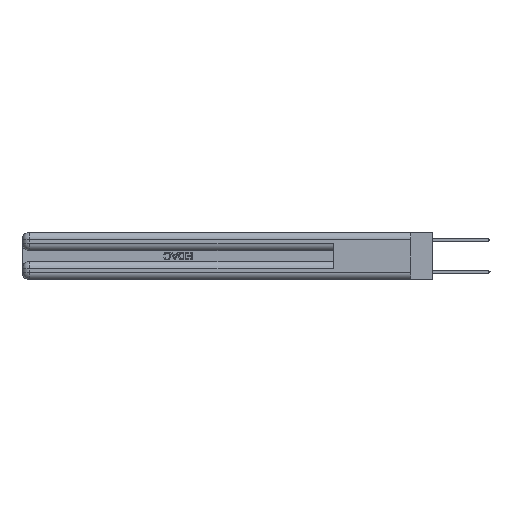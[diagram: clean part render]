
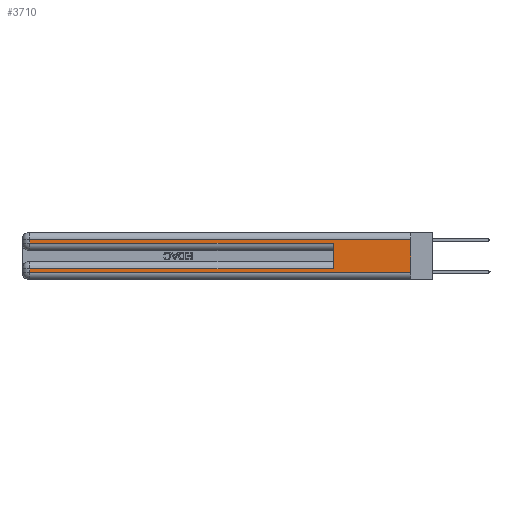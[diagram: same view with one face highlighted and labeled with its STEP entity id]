
A CAD part, left-side view. The second image highlights one B-rep face of the part: STEP entity #3710.
In plain terms, the highlighted planar face has unit normal (-1, 0, 0).
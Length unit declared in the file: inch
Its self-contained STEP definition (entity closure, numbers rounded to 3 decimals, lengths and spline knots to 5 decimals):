
#791 = EDGE_CURVE ( 'NONE', #13586, #18417, #19519, .T. ) ;
#1334 = CARTESIAN_POINT ( 'NONE',  ( 0., 2.94, 0.37 ) ) ;
#1484 = VECTOR ( 'NONE', #6819, 39.37008 ) ;
#2397 = PLANE ( 'NONE',  #27314 ) ;
#2539 = VECTOR ( 'NONE', #17491, 39.37008 ) ;
#3710 = ADVANCED_FACE ( 'NONE', ( #32501 ), #2397, .F. ) ;
#4244 = VERTEX_POINT ( 'NONE', #26098 ) ;
#4618 = ORIENTED_EDGE ( 'NONE', *, *, #24827, .T. ) ;
#5021 = ORIENTED_EDGE ( 'NONE', *, *, #18827, .T. ) ;
#5046 = VECTOR ( 'NONE', #24689, 39.37008 ) ;
#5087 = CARTESIAN_POINT ( 'NONE',  ( 0., 0., 0.37 ) ) ;
#5251 = VECTOR ( 'NONE', #16092, 39.37008 ) ;
#5774 = ORIENTED_EDGE ( 'NONE', *, *, #29402, .F. ) ;
#5963 = ORIENTED_EDGE ( 'NONE', *, *, #29117, .T. ) ;
#6102 = CARTESIAN_POINT ( 'NONE',  ( 0., 0., 0.285 ) ) ;
#6352 = VECTOR ( 'NONE', #8772, 39.37008 ) ;
#6819 = DIRECTION ( 'NONE',  ( 0., 0., -1. ) ) ;
#7538 = CARTESIAN_POINT ( 'NONE',  ( 0., 0., 0.06 ) ) ;
#7709 = ORIENTED_EDGE ( 'NONE', *, *, #9601, .T. ) ;
#7748 = CARTESIAN_POINT ( 'NONE',  ( 0., 0.6, 0.285 ) ) ;
#7762 = DIRECTION ( 'NONE',  ( 0., 0., -1. ) ) ;
#8162 = DIRECTION ( 'NONE',  ( 0., 0., 1. ) ) ;
#8569 = LINE ( 'NONE', #1334, #1484 ) ;
#8772 = DIRECTION ( 'NONE',  ( 0., -1., 0. ) ) ;
#8847 = CARTESIAN_POINT ( 'NONE',  ( 0., 0., 0.31 ) ) ;
#8966 = VECTOR ( 'NONE', #30380, 39.37008 ) ;
#9601 = EDGE_CURVE ( 'NONE', #30058, #17965, #8569, .T. ) ;
#9662 = LINE ( 'NONE', #27959, #2539 ) ;
#10101 = ORIENTED_EDGE ( 'NONE', *, *, #791, .F. ) ;
#10317 = ORIENTED_EDGE ( 'NONE', *, *, #25605, .T. ) ;
#10763 = CARTESIAN_POINT ( 'NONE',  ( 0., 0., 0.085 ) ) ;
#10765 = VERTEX_POINT ( 'NONE', #7538 ) ;
#10794 = DIRECTION ( 'NONE',  ( 0., 0., -1. ) ) ;
#11095 = CARTESIAN_POINT ( 'NONE',  ( 0., 0.6, 0.085 ) ) ;
#12100 = CARTESIAN_POINT ( 'NONE',  ( 0., 2.94, 0.31 ) ) ;
#12458 = VECTOR ( 'NONE', #8162, 39.37008 ) ;
#12657 = LINE ( 'NONE', #23965, #26691 ) ;
#13227 = CARTESIAN_POINT ( 'NONE',  ( 0., 2.94, 0.085 ) ) ;
#13402 = LINE ( 'NONE', #6102, #6352 ) ;
#13586 = VERTEX_POINT ( 'NONE', #11095 ) ;
#13772 = LINE ( 'NONE', #8847, #5046 ) ;
#16092 = DIRECTION ( 'NONE',  ( 0., 1., 0. ) ) ;
#17491 = DIRECTION ( 'NONE',  ( 0., -1., 0. ) ) ;
#17965 = VERTEX_POINT ( 'NONE', #26971 ) ;
#18017 = CARTESIAN_POINT ( 'NONE',  ( 0., 0., 0.31 ) ) ;
#18417 = VERTEX_POINT ( 'NONE', #7748 ) ;
#18827 = EDGE_CURVE ( 'NONE', #4244, #10765, #9662, .T. ) ;
#18851 = CARTESIAN_POINT ( 'NONE',  ( 0., 0.6, 0.145 ) ) ;
#19519 = LINE ( 'NONE', #18851, #12458 ) ;
#21656 = ORIENTED_EDGE ( 'NONE', *, *, #24171, .T. ) ;
#22458 = EDGE_LOOP ( 'NONE', ( #5774, #10317, #7709, #4618, #10101, #5963, #21656, #5021 ) ) ;
#23620 = DIRECTION ( 'NONE',  ( 1., 0., 0. ) ) ;
#23965 = CARTESIAN_POINT ( 'NONE',  ( 0., 2.94, 0.37 ) ) ;
#24171 = EDGE_CURVE ( 'NONE', #30370, #4244, #12657, .T. ) ;
#24689 = DIRECTION ( 'NONE',  ( 0., 1., 0. ) ) ;
#24827 = EDGE_CURVE ( 'NONE', #17965, #18417, #13402, .T. ) ;
#25061 = CARTESIAN_POINT ( 'NONE',  ( 0., 0., 0.37 ) ) ;
#25605 = EDGE_CURVE ( 'NONE', #27396, #30058, #13772, .T. ) ;
#26098 = CARTESIAN_POINT ( 'NONE',  ( 0., 2.94, 0.06 ) ) ;
#26691 = VECTOR ( 'NONE', #10794, 39.37008 ) ;
#26971 = CARTESIAN_POINT ( 'NONE',  ( 0., 2.94, 0.285 ) ) ;
#27314 = AXIS2_PLACEMENT_3D ( 'NONE', #5087, #23620, #7762 ) ;
#27396 = VERTEX_POINT ( 'NONE', #18017 ) ;
#27959 = CARTESIAN_POINT ( 'NONE',  ( 0., 0., 0.06 ) ) ;
#29117 = EDGE_CURVE ( 'NONE', #13586, #30370, #32564, .T. ) ;
#29216 = LINE ( 'NONE', #25061, #8966 ) ;
#29402 = EDGE_CURVE ( 'NONE', #27396, #10765, #29216, .T. ) ;
#30058 = VERTEX_POINT ( 'NONE', #12100 ) ;
#30370 = VERTEX_POINT ( 'NONE', #13227 ) ;
#30380 = DIRECTION ( 'NONE',  ( 0., 0., -1. ) ) ;
#32501 = FACE_OUTER_BOUND ( 'NONE', #22458, .T. ) ;
#32564 = LINE ( 'NONE', #10763, #5251 ) ;
